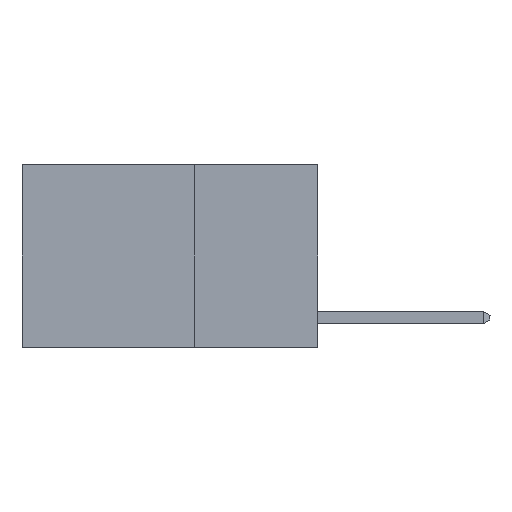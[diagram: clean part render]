
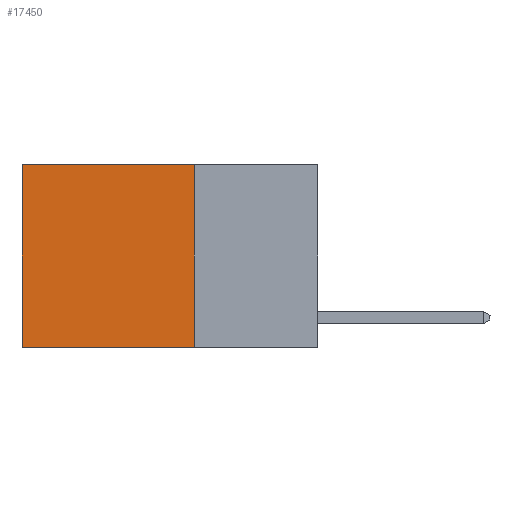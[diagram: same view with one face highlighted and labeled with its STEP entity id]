
A CAD part, left-side view. The second image highlights one B-rep face of the part: STEP entity #17450.
In plain terms, the highlighted planar face has unit normal (-1, 0, 0).
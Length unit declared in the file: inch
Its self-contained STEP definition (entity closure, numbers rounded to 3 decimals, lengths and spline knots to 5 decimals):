
#75 = VECTOR ( 'NONE', #6681, 39.37008 ) ;
#355 = VECTOR ( 'NONE', #14653, 39.37008 ) ;
#665 = CARTESIAN_POINT ( 'NONE',  ( 0.2625, 0.25, 0. ) ) ;
#689 = LINE ( 'NONE', #1164, #75 ) ;
#1164 = CARTESIAN_POINT ( 'NONE',  ( 0.2625, 0.6, 0. ) ) ;
#1383 = EDGE_CURVE ( 'NONE', #1589, #19178, #21466, .T. ) ;
#1396 = EDGE_CURVE ( 'NONE', #19178, #11271, #16409, .T. ) ;
#1538 = DIRECTION ( 'NONE',  ( 0., 1., 0. ) ) ;
#1589 = VERTEX_POINT ( 'NONE', #665 ) ;
#3213 = VECTOR ( 'NONE', #1538, 39.37008 ) ;
#3349 = DIRECTION ( 'NONE',  ( 0., 0., -1. ) ) ;
#3745 = DIRECTION ( 'NONE',  ( 1., 0., 0. ) ) ;
#5995 = EDGE_CURVE ( 'NONE', #1589, #10842, #22292, .T. ) ;
#6681 = DIRECTION ( 'NONE',  ( 0., 0., -1. ) ) ;
#6935 = CARTESIAN_POINT ( 'NONE',  ( 0.2625, 0.25, -0.37 ) ) ;
#7146 = AXIS2_PLACEMENT_3D ( 'NONE', #20081, #3745, #3349 ) ;
#9091 = CARTESIAN_POINT ( 'NONE',  ( 0.2625, 0.25, 0. ) ) ;
#9113 = CARTESIAN_POINT ( 'NONE',  ( 0.2625, 0.25, -0.37 ) ) ;
#10296 = CARTESIAN_POINT ( 'NONE',  ( 0.2625, 0.25, 0. ) ) ;
#10842 = VERTEX_POINT ( 'NONE', #22530 ) ;
#11271 = VERTEX_POINT ( 'NONE', #11808 ) ;
#11460 = ORIENTED_EDGE ( 'NONE', *, *, #1383, .F. ) ;
#11808 = CARTESIAN_POINT ( 'NONE',  ( 0.2625, 0.6, -0.37 ) ) ;
#14170 = VECTOR ( 'NONE', #17761, 39.37008 ) ;
#14653 = DIRECTION ( 'NONE',  ( 0., 1., 0. ) ) ;
#15008 = FACE_OUTER_BOUND ( 'NONE', #18055, .T. ) ;
#16409 = LINE ( 'NONE', #6935, #355 ) ;
#17224 = ORIENTED_EDGE ( 'NONE', *, *, #23430, .T. ) ;
#17450 = ADVANCED_FACE ( 'NONE', ( #15008 ), #22497, .F. ) ;
#17761 = DIRECTION ( 'NONE',  ( 0., 0., -1. ) ) ;
#17987 = ORIENTED_EDGE ( 'NONE', *, *, #1396, .F. ) ;
#18055 = EDGE_LOOP ( 'NONE', ( #17224, #17987, #11460, #20263 ) ) ;
#19178 = VERTEX_POINT ( 'NONE', #9113 ) ;
#20081 = CARTESIAN_POINT ( 'NONE',  ( 0.2625, 0.25, 0. ) ) ;
#20263 = ORIENTED_EDGE ( 'NONE', *, *, #5995, .T. ) ;
#21466 = LINE ( 'NONE', #10296, #14170 ) ;
#22292 = LINE ( 'NONE', #9091, #3213 ) ;
#22497 = PLANE ( 'NONE',  #7146 ) ;
#22530 = CARTESIAN_POINT ( 'NONE',  ( 0.2625, 0.6, 0. ) ) ;
#23430 = EDGE_CURVE ( 'NONE', #10842, #11271, #689, .T. ) ;
